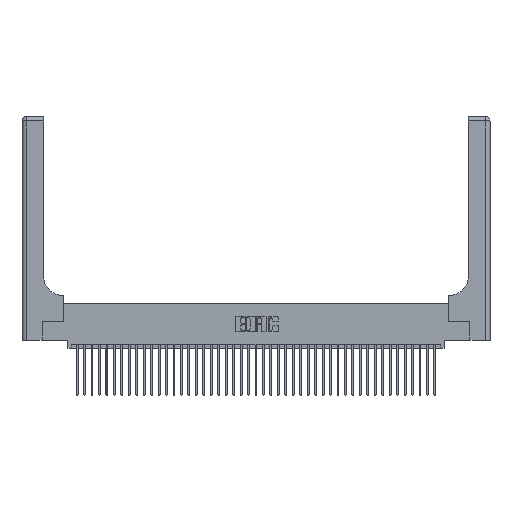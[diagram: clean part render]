
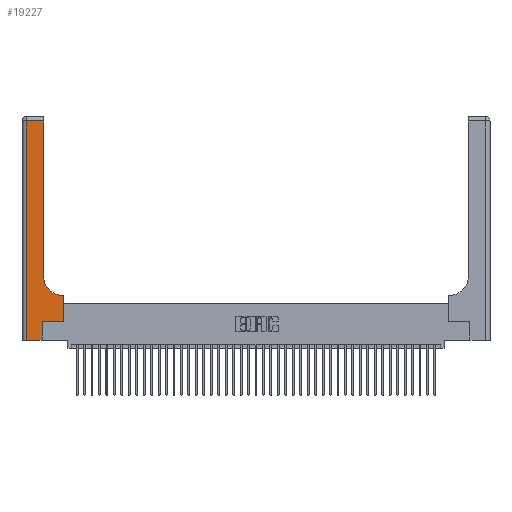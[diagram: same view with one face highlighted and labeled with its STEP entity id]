
A CAD part, top view. The second image highlights one B-rep face of the part: STEP entity #19227.
In plain terms, the highlighted planar face has unit normal (0, 0, 1).
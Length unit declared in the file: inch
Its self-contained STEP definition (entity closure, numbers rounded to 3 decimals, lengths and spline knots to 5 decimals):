
#97 = LINE ( 'NONE', #13338, #34251 ) ;
#358 = ORIENTED_EDGE ( 'NONE', *, *, #30544, .T. ) ;
#457 = CARTESIAN_POINT ( 'NONE',  ( 0.2915, 2.94, 0.37 ) ) ;
#997 = CARTESIAN_POINT ( 'NONE',  ( 0.269, 0.25, 0.37 ) ) ;
#1040 = CARTESIAN_POINT ( 'NONE',  ( 0., 0., 0.37 ) ) ;
#2424 = LINE ( 'NONE', #42211, #26701 ) ;
#2431 = CARTESIAN_POINT ( 'NONE',  ( 0., 3., 0.37 ) ) ;
#2623 = DIRECTION ( 'NONE',  ( -1., 0., 0. ) ) ;
#3367 = CARTESIAN_POINT ( 'NONE',  ( 0.5415, 0.85, 0.37 ) ) ;
#3459 = VERTEX_POINT ( 'NONE', #457 ) ;
#3924 = EDGE_CURVE ( 'NONE', #20433, #42162, #28604, .T. ) ;
#3982 = DIRECTION ( 'NONE',  ( 0., 1., 0. ) ) ;
#5886 = LINE ( 'NONE', #13906, #32240 ) ;
#6435 = VECTOR ( 'NONE', #35915, 39.37008 ) ;
#6692 = DIRECTION ( 'NONE',  ( 1., 0., 0. ) ) ;
#7450 = VERTEX_POINT ( 'NONE', #26952 ) ;
#7830 = VECTOR ( 'NONE', #32177, 39.37008 ) ;
#9235 = DIRECTION ( 'NONE',  ( 0., 0., -1. ) ) ;
#9880 = AXIS2_PLACEMENT_3D ( 'NONE', #2431, #9235, #32358 ) ;
#10145 = ORIENTED_EDGE ( 'NONE', *, *, #41742, .T. ) ;
#10301 = FACE_OUTER_BOUND ( 'NONE', #42274, .T. ) ;
#12299 = VERTEX_POINT ( 'NONE', #997 ) ;
#13338 = CARTESIAN_POINT ( 'NONE',  ( 0.5585, 0.25, 0.37 ) ) ;
#13906 = CARTESIAN_POINT ( 'NONE',  ( 0.2915, 3., 0.37 ) ) ;
#14382 = EDGE_CURVE ( 'NONE', #37690, #42092, #36134, .T. ) ;
#15484 = CARTESIAN_POINT ( 'NONE',  ( 0., 2.94, 0.37 ) ) ;
#16683 = DIRECTION ( 'NONE',  ( 0., 1., 0. ) ) ;
#18254 = EDGE_CURVE ( 'NONE', #3459, #34572, #36769, .T. ) ;
#18414 = CARTESIAN_POINT ( 'NONE',  ( 0.06, 2.94, 0.37 ) ) ;
#18980 = ORIENTED_EDGE ( 'NONE', *, *, #18254, .T. ) ;
#19227 = ADVANCED_FACE ( 'NONE', ( #10301 ), #28994, .F. ) ;
#19899 = CARTESIAN_POINT ( 'NONE',  ( 0.5585, 0.6, 0.37 ) ) ;
#20433 = VERTEX_POINT ( 'NONE', #38956 ) ;
#20838 = DIRECTION ( 'NONE',  ( 1., 0., 0. ) ) ;
#22286 = EDGE_CURVE ( 'NONE', #42092, #12299, #40550, .T. ) ;
#22536 = EDGE_CURVE ( 'NONE', #42162, #3459, #5886, .T. ) ;
#26425 = DIRECTION ( 'NONE',  ( 0., 0., -1. ) ) ;
#26701 = VECTOR ( 'NONE', #2623, 39.37008 ) ;
#26914 = ORIENTED_EDGE ( 'NONE', *, *, #22286, .T. ) ;
#26952 = CARTESIAN_POINT ( 'NONE',  ( 0.5585, 0.25, 0.37 ) ) ;
#27299 = VECTOR ( 'NONE', #20838, 39.37008 ) ;
#27456 = LINE ( 'NONE', #35363, #7830 ) ;
#28060 = ORIENTED_EDGE ( 'NONE', *, *, #32260, .T. ) ;
#28604 = CIRCLE ( 'NONE', #39055, 0.25 ) ;
#28994 = PLANE ( 'NONE',  #9880 ) ;
#29316 = DIRECTION ( 'NONE',  ( 1., 0., 0. ) ) ;
#29963 = EDGE_CURVE ( 'NONE', #7450, #34271, #97, .T. ) ;
#30544 = EDGE_CURVE ( 'NONE', #12299, #7450, #32156, .T. ) ;
#31197 = CARTESIAN_POINT ( 'NONE',  ( 0.269, 0., 0.37 ) ) ;
#31307 = CARTESIAN_POINT ( 'NONE',  ( 0.06, 0., 0.37 ) ) ;
#32156 = LINE ( 'NONE', #39345, #33199 ) ;
#32177 = DIRECTION ( 'NONE',  ( 0., -1., 0. ) ) ;
#32240 = VECTOR ( 'NONE', #3982, 39.37008 ) ;
#32260 = EDGE_CURVE ( 'NONE', #34572, #37690, #27456, .T. ) ;
#32358 = DIRECTION ( 'NONE',  ( -1., 0., 0. ) ) ;
#33199 = VECTOR ( 'NONE', #29316, 39.37008 ) ;
#34151 = ORIENTED_EDGE ( 'NONE', *, *, #22536, .T. ) ;
#34251 = VECTOR ( 'NONE', #16683, 39.37008 ) ;
#34271 = VERTEX_POINT ( 'NONE', #19899 ) ;
#34572 = VERTEX_POINT ( 'NONE', #18414 ) ;
#34877 = ORIENTED_EDGE ( 'NONE', *, *, #3924, .T. ) ;
#34939 = CARTESIAN_POINT ( 'NONE',  ( 0.2915, 0.85, 0.37 ) ) ;
#35173 = ORIENTED_EDGE ( 'NONE', *, *, #14382, .T. ) ;
#35363 = CARTESIAN_POINT ( 'NONE',  ( 0.06, 3., 0.37 ) ) ;
#35915 = DIRECTION ( 'NONE',  ( 0., 1., 0. ) ) ;
#36134 = LINE ( 'NONE', #1040, #27299 ) ;
#36769 = LINE ( 'NONE', #15484, #38857 ) ;
#37690 = VERTEX_POINT ( 'NONE', #31307 ) ;
#38623 = DIRECTION ( 'NONE',  ( -1., 0., 0. ) ) ;
#38857 = VECTOR ( 'NONE', #38623, 39.37008 ) ;
#38956 = CARTESIAN_POINT ( 'NONE',  ( 0.5415, 0.6, 0.37 ) ) ;
#39055 = AXIS2_PLACEMENT_3D ( 'NONE', #3367, #26425, #6692 ) ;
#39116 = CARTESIAN_POINT ( 'NONE',  ( 0.269, 0., 0.37 ) ) ;
#39345 = CARTESIAN_POINT ( 'NONE',  ( 0.269, 0.25, 0.37 ) ) ;
#40048 = ORIENTED_EDGE ( 'NONE', *, *, #29963, .T. ) ;
#40550 = LINE ( 'NONE', #39116, #6435 ) ;
#41742 = EDGE_CURVE ( 'NONE', #34271, #20433, #2424, .T. ) ;
#42092 = VERTEX_POINT ( 'NONE', #31197 ) ;
#42162 = VERTEX_POINT ( 'NONE', #34939 ) ;
#42211 = CARTESIAN_POINT ( 'NONE',  ( 0.2915, 0.6, 0.37 ) ) ;
#42274 = EDGE_LOOP ( 'NONE', ( #34151, #18980, #28060, #35173, #26914, #358, #40048, #10145, #34877 ) ) ;
